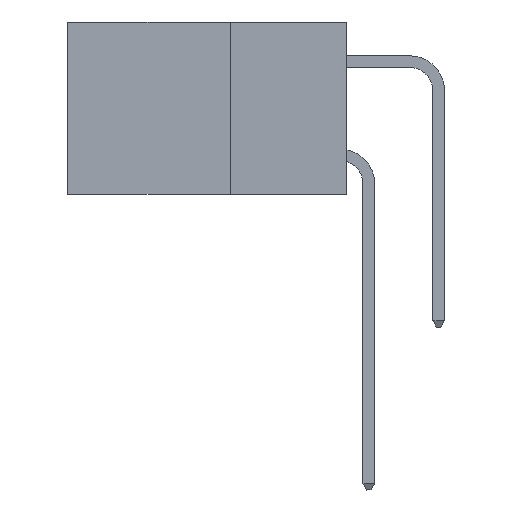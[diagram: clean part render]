
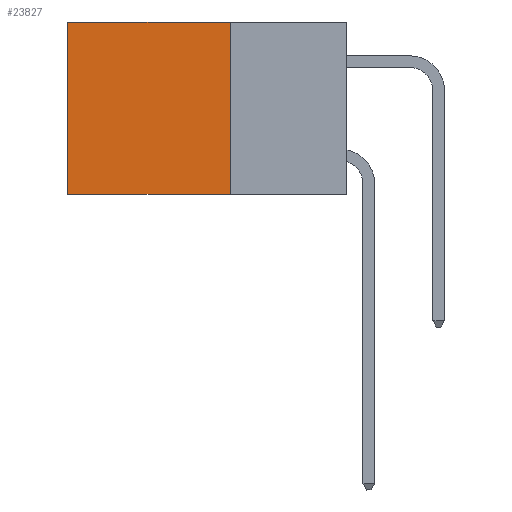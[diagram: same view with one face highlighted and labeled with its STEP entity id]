
A CAD part, left-side view. The second image highlights one B-rep face of the part: STEP entity #23827.
In plain terms, the highlighted planar face has unit normal (-1, 0, 0).
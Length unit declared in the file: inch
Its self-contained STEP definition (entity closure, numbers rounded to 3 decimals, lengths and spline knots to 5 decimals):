
#591 = DIRECTION ( 'NONE',  ( 0., 0., -1. ) ) ;
#1178 = DIRECTION ( 'NONE',  ( 0., 1., 0. ) ) ;
#2630 = VERTEX_POINT ( 'NONE', #5744 ) ;
#3645 = LINE ( 'NONE', #20599, #20266 ) ;
#3864 = ORIENTED_EDGE ( 'NONE', *, *, #25131, .T. ) ;
#4457 = DIRECTION ( 'NONE',  ( 0., 1., 0. ) ) ;
#5168 = EDGE_CURVE ( 'NONE', #7828, #2630, #3645, .T. ) ;
#5744 = CARTESIAN_POINT ( 'NONE',  ( 0.2875, 0.6, -0.37 ) ) ;
#7355 = CARTESIAN_POINT ( 'NONE',  ( 0.2875, 0.25, 0. ) ) ;
#7541 = VECTOR ( 'NONE', #1178, 39.37008 ) ;
#7828 = VERTEX_POINT ( 'NONE', #12006 ) ;
#8341 = CARTESIAN_POINT ( 'NONE',  ( 0.2875, 0.25, 0. ) ) ;
#9929 = DIRECTION ( 'NONE',  ( 0., 0., -1. ) ) ;
#11159 = DIRECTION ( 'NONE',  ( 0., 0., -1. ) ) ;
#11702 = LINE ( 'NONE', #7355, #23044 ) ;
#12006 = CARTESIAN_POINT ( 'NONE',  ( 0.2875, 0.6, 0. ) ) ;
#12623 = AXIS2_PLACEMENT_3D ( 'NONE', #19705, #23935, #11159 ) ;
#13197 = CARTESIAN_POINT ( 'NONE',  ( 0.2875, 0.25, 0. ) ) ;
#13895 = EDGE_LOOP ( 'NONE', ( #16210, #14793, #19114, #3864 ) ) ;
#14793 = ORIENTED_EDGE ( 'NONE', *, *, #26099, .F. ) ;
#15155 = EDGE_CURVE ( 'NONE', #21489, #23233, #11702, .T. ) ;
#16210 = ORIENTED_EDGE ( 'NONE', *, *, #5168, .T. ) ;
#18685 = CARTESIAN_POINT ( 'NONE',  ( 0.2875, 0.25, -0.37 ) ) ;
#19016 = LINE ( 'NONE', #18685, #7541 ) ;
#19114 = ORIENTED_EDGE ( 'NONE', *, *, #15155, .F. ) ;
#19513 = FACE_OUTER_BOUND ( 'NONE', #13895, .T. ) ;
#19705 = CARTESIAN_POINT ( 'NONE',  ( 0.2875, 0.25, 0. ) ) ;
#20266 = VECTOR ( 'NONE', #9929, 39.37008 ) ;
#20599 = CARTESIAN_POINT ( 'NONE',  ( 0.2875, 0.6, 0. ) ) ;
#21489 = VERTEX_POINT ( 'NONE', #8341 ) ;
#21683 = VECTOR ( 'NONE', #4457, 39.37008 ) ;
#22831 = CARTESIAN_POINT ( 'NONE',  ( 0.2875, 0.25, -0.37 ) ) ;
#23044 = VECTOR ( 'NONE', #591, 39.37008 ) ;
#23233 = VERTEX_POINT ( 'NONE', #22831 ) ;
#23827 = ADVANCED_FACE ( 'NONE', ( #19513 ), #25982, .F. ) ;
#23935 = DIRECTION ( 'NONE',  ( 1., 0., 0. ) ) ;
#25131 = EDGE_CURVE ( 'NONE', #21489, #7828, #27991, .T. ) ;
#25982 = PLANE ( 'NONE',  #12623 ) ;
#26099 = EDGE_CURVE ( 'NONE', #23233, #2630, #19016, .T. ) ;
#27991 = LINE ( 'NONE', #13197, #21683 ) ;
